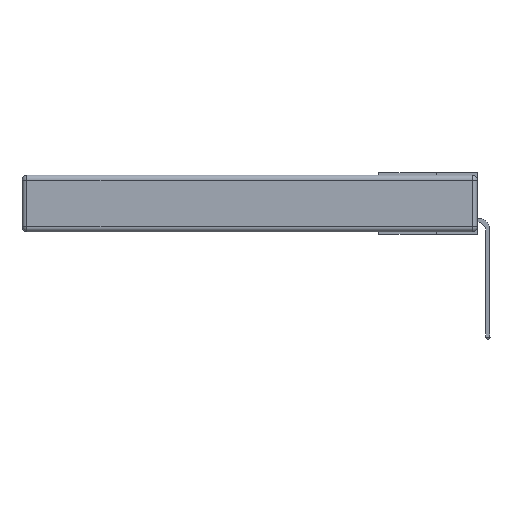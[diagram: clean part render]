
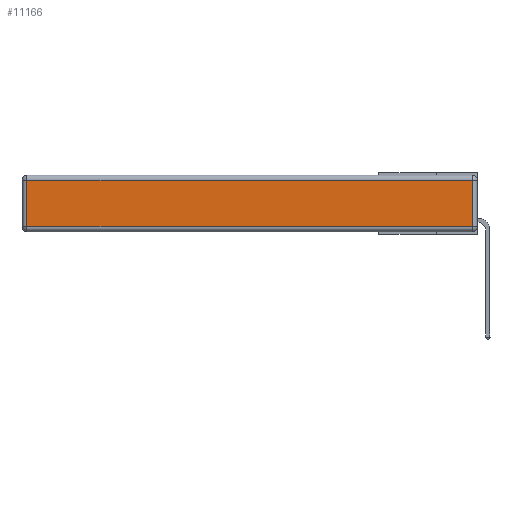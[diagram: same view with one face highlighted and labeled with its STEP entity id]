
A CAD part, left-side view. The second image highlights one B-rep face of the part: STEP entity #11166.
In plain terms, the highlighted planar face has unit normal (-1, 0, 0).
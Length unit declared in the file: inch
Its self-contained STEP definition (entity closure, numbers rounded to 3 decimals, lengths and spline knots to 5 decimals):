
#18 = VERTEX_POINT ( 'NONE', #9378 ) ;
#140 = ORIENTED_EDGE ( 'NONE', *, *, #7216, .T. ) ;
#691 = EDGE_CURVE ( 'NONE', #4820, #18, #8651, .T. ) ;
#717 = LINE ( 'NONE', #3684, #8894 ) ;
#988 = DIRECTION ( 'NONE',  ( 0., 1., 0. ) ) ;
#2457 = EDGE_CURVE ( 'NONE', #10906, #4820, #10918, .T. ) ;
#2564 = VECTOR ( 'NONE', #9606, 39.37008 ) ;
#3190 = ORIENTED_EDGE ( 'NONE', *, *, #2457, .T. ) ;
#3313 = VERTEX_POINT ( 'NONE', #7344 ) ;
#3684 = CARTESIAN_POINT ( 'NONE',  ( 0., 2.72, -0.343 ) ) ;
#4152 = VECTOR ( 'NONE', #988, 39.37008 ) ;
#4357 = CARTESIAN_POINT ( 'NONE',  ( 0., 0.03, -0.343 ) ) ;
#4367 = CARTESIAN_POINT ( 'NONE',  ( 0., 2.75, -0.03 ) ) ;
#4461 = LINE ( 'NONE', #12076, #11940 ) ;
#4820 = VERTEX_POINT ( 'NONE', #11950 ) ;
#4878 = DIRECTION ( 'NONE',  ( 0., -1., 0. ) ) ;
#5499 = EDGE_LOOP ( 'NONE', ( #12391, #3190, #13615, #140 ) ) ;
#6289 = AXIS2_PLACEMENT_3D ( 'NONE', #10285, #8066, #11355 ) ;
#6635 = FACE_OUTER_BOUND ( 'NONE', #5499, .T. ) ;
#7216 = EDGE_CURVE ( 'NONE', #18, #3313, #717, .T. ) ;
#7344 = CARTESIAN_POINT ( 'NONE',  ( 0., 2.72, -0.313 ) ) ;
#8011 = DIRECTION ( 'NONE',  ( 0., 0., -1. ) ) ;
#8066 = DIRECTION ( 'NONE',  ( -1., 0., 0. ) ) ;
#8651 = LINE ( 'NONE', #4367, #4152 ) ;
#8894 = VECTOR ( 'NONE', #8011, 39.37008 ) ;
#9378 = CARTESIAN_POINT ( 'NONE',  ( 0., 2.72, -0.03 ) ) ;
#9606 = DIRECTION ( 'NONE',  ( 0., 0., 1. ) ) ;
#9967 = CARTESIAN_POINT ( 'NONE',  ( 0., 0.03, -0.313 ) ) ;
#10285 = CARTESIAN_POINT ( 'NONE',  ( 0., 0., -0.343 ) ) ;
#10906 = VERTEX_POINT ( 'NONE', #9967 ) ;
#10918 = LINE ( 'NONE', #4357, #2564 ) ;
#11166 = ADVANCED_FACE ( 'NONE', ( #6635 ), #13464, .T. ) ;
#11355 = DIRECTION ( 'NONE',  ( 0., 0., 1. ) ) ;
#11940 = VECTOR ( 'NONE', #4878, 39.37008 ) ;
#11950 = CARTESIAN_POINT ( 'NONE',  ( 0., 0.03, -0.03 ) ) ;
#12076 = CARTESIAN_POINT ( 'NONE',  ( 0., 0., -0.313 ) ) ;
#12391 = ORIENTED_EDGE ( 'NONE', *, *, #12885, .T. ) ;
#12885 = EDGE_CURVE ( 'NONE', #3313, #10906, #4461, .T. ) ;
#13464 = PLANE ( 'NONE',  #6289 ) ;
#13615 = ORIENTED_EDGE ( 'NONE', *, *, #691, .T. ) ;
